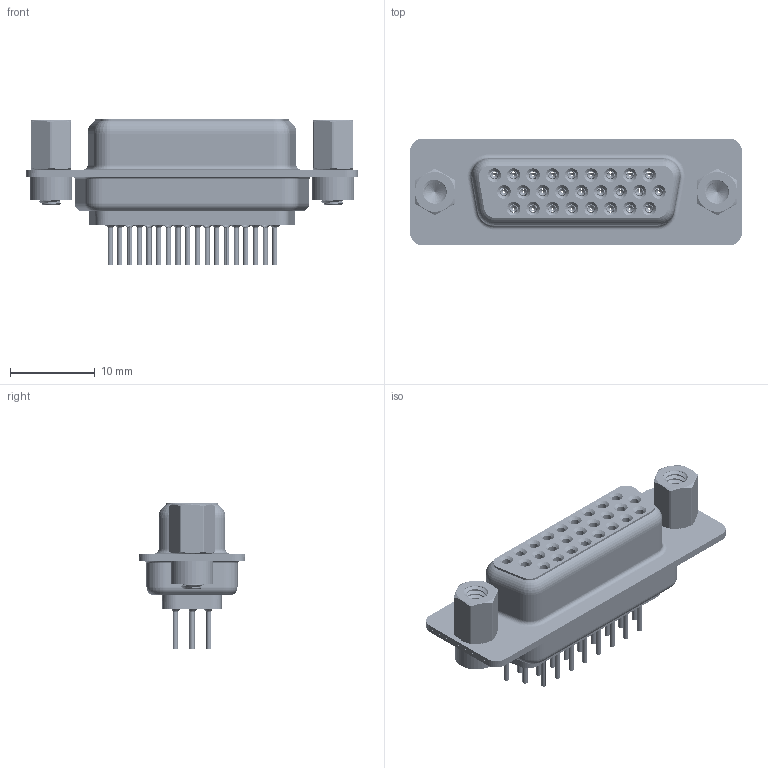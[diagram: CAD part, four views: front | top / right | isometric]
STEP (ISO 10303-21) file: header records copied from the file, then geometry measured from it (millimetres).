
FILE_DESCRIPTION (( 'STEP AP203' ), '1' );
FILE_NAME ('638-026-330-243.STEP', '2020-07-18T20:28:07', ( '' ), ( '' ), 'SwSTEP 2.0', 'SolidWorks 2020', '' );
FILE_SCHEMA (( 'CONFIG_CONTROL_DESIGN' ));
Length unit declared in the file: millimetre
Products named in the file (9): 638 Housing_26 Contacts; 638 Contact Row 3_30; 638 4-40 Threaded Rivet; 638-026-330-243; 638 Contact Row 1_30; 638 4-40 Hex Standoff; 638 Shell Front_26 Contacts; 638 Shell Rear_26 Contacts; 638 Contact Row 2_30
Assembly tree (33 placements, depth 2):
  638-026-330-243
    638 Housing_26 Contacts
    638 Shell Front_26 Contacts
    638 Shell Rear_26 Contacts
    638 Contact Row 1_30  x9
    638 Contact Row 2_30  x9
    638 Contact Row 3_30  x8
    638 4-40 Threaded Rivet  x2
    638 4-40 Hex Standoff  x2
Bounding box: 39.19 x 12.6 x 17.3 mm (x, y, z)
Volume: 2426.1 mm3; surface area: 8790 mm2
Topology: 33 solids, 33 shells, 3707 faces, 9457 edges, 5879 vertices
Faces by surface type: cylinder 1067, plane 895, torus 733, bspline 538, cone 474
Entity records: 37509 total; most frequent: CARTESIAN_POINT 12993, DIRECTION 4907, ORIENTED_EDGE 4754, EDGE_CURVE 2377, AXIS2_PLACEMENT_3D 2045, VERTEX_POINT 1499, EDGE_LOOP 1138, CIRCLE 1095
